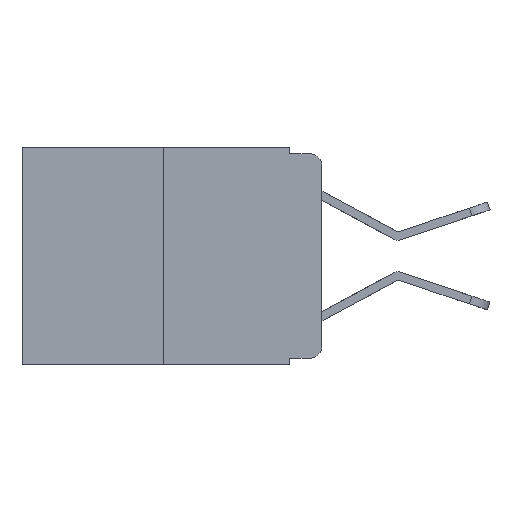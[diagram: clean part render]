
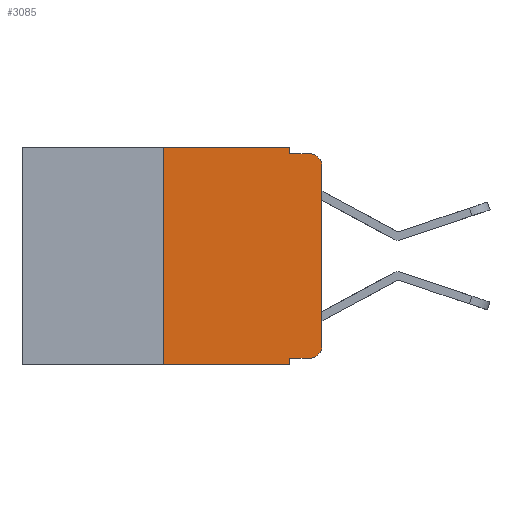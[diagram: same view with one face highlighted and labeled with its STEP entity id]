
A CAD part, left-side view. The second image highlights one B-rep face of the part: STEP entity #3085.
In plain terms, the highlighted planar face has unit normal (-1, 0, 0).
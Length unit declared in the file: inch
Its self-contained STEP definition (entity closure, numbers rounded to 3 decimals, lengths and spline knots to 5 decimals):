
#28 = VERTEX_POINT ( 'NONE', #774 ) ;
#284 = VECTOR ( 'NONE', #11346, 39.37008 ) ;
#288 = CARTESIAN_POINT ( 'NONE',  ( 0., 0.051, 0. ) ) ;
#741 = DIRECTION ( 'NONE',  ( 0., 0., 1. ) ) ;
#774 = CARTESIAN_POINT ( 'NONE',  ( 0., 0.051, 0. ) ) ;
#978 = CARTESIAN_POINT ( 'NONE',  ( 0., 0., -0.03 ) ) ;
#1115 = CARTESIAN_POINT ( 'NONE',  ( 0., 0.02, -0.333 ) ) ;
#1188 = VERTEX_POINT ( 'NONE', #10671 ) ;
#1215 = CARTESIAN_POINT ( 'NONE',  ( 0., 0.051, -0.333 ) ) ;
#1330 = VERTEX_POINT ( 'NONE', #1115 ) ;
#1332 = LINE ( 'NONE', #7927, #8927 ) ;
#1438 = VERTEX_POINT ( 'NONE', #9221 ) ;
#1450 = VERTEX_POINT ( 'NONE', #4686 ) ;
#1580 = EDGE_CURVE ( 'NONE', #1450, #4527, #5750, .T. ) ;
#1722 = AXIS2_PLACEMENT_3D ( 'NONE', #4035, #10585, #5033 ) ;
#1853 = ORIENTED_EDGE ( 'NONE', *, *, #3724, .F. ) ;
#2213 = ORIENTED_EDGE ( 'NONE', *, *, #10275, .T. ) ;
#2307 = EDGE_CURVE ( 'NONE', #28, #1188, #2885, .T. ) ;
#2504 = EDGE_CURVE ( 'NONE', #1450, #8013, #1332, .T. ) ;
#2551 = DIRECTION ( 'NONE',  ( 0., 0., -1. ) ) ;
#2592 = DIRECTION ( 'NONE',  ( 1., 0., 0. ) ) ;
#2665 = VERTEX_POINT ( 'NONE', #11396 ) ;
#2686 = ORIENTED_EDGE ( 'NONE', *, *, #12070, .F. ) ;
#2885 = LINE ( 'NONE', #288, #284 ) ;
#3085 = ADVANCED_FACE ( 'NONE', ( #10567 ), #5547, .F. ) ;
#3231 = CARTESIAN_POINT ( 'NONE',  ( 0., 0.051, 0. ) ) ;
#3233 = CARTESIAN_POINT ( 'NONE',  ( 0., 0.25, 0. ) ) ;
#3294 = ORIENTED_EDGE ( 'NONE', *, *, #2307, .F. ) ;
#3724 = EDGE_CURVE ( 'NONE', #1188, #1438, #7327, .T. ) ;
#3977 = VECTOR ( 'NONE', #741, 39.37008 ) ;
#4012 = CARTESIAN_POINT ( 'NONE',  ( 0., 0.473, 0. ) ) ;
#4035 = CARTESIAN_POINT ( 'NONE',  ( 0., 0.02, -0.313 ) ) ;
#4527 = VERTEX_POINT ( 'NONE', #4533 ) ;
#4533 = CARTESIAN_POINT ( 'NONE',  ( 0., 0.25, 0. ) ) ;
#4546 = LINE ( 'NONE', #1215, #9278 ) ;
#4592 = DIRECTION ( 'NONE',  ( 0., -1., 0. ) ) ;
#4686 = CARTESIAN_POINT ( 'NONE',  ( 0., 0.25, -0.343 ) ) ;
#4696 = LINE ( 'NONE', #9319, #11775 ) ;
#4878 = DIRECTION ( 'NONE',  ( 0., -1., 0. ) ) ;
#4960 = CARTESIAN_POINT ( 'NONE',  ( 0., 0., 0. ) ) ;
#5033 = DIRECTION ( 'NONE',  ( 0., 0., -1. ) ) ;
#5062 = EDGE_CURVE ( 'NONE', #6580, #1438, #5335, .T. ) ;
#5335 = CIRCLE ( 'NONE', #5743, 0.02 ) ;
#5495 = CIRCLE ( 'NONE', #1722, 0.02 ) ;
#5547 = PLANE ( 'NONE',  #9251 ) ;
#5743 = AXIS2_PLACEMENT_3D ( 'NONE', #8003, #7967, #10916 ) ;
#5750 = LINE ( 'NONE', #3233, #6346 ) ;
#6269 = CARTESIAN_POINT ( 'NONE',  ( 0., 0.051, -0.333 ) ) ;
#6346 = VECTOR ( 'NONE', #7991, 39.37008 ) ;
#6372 = EDGE_CURVE ( 'NONE', #2665, #6580, #11141, .T. ) ;
#6580 = VERTEX_POINT ( 'NONE', #978 ) ;
#7327 = LINE ( 'NONE', #12593, #7898 ) ;
#7340 = EDGE_LOOP ( 'NONE', ( #12009, #8517, #1853, #3294, #7661, #12170, #7346, #2686, #10999, #2213 ) ) ;
#7346 = ORIENTED_EDGE ( 'NONE', *, *, #2504, .T. ) ;
#7661 = ORIENTED_EDGE ( 'NONE', *, *, #10975, .F. ) ;
#7898 = VECTOR ( 'NONE', #4878, 39.37008 ) ;
#7927 = CARTESIAN_POINT ( 'NONE',  ( 0., 0.473, -0.343 ) ) ;
#7967 = DIRECTION ( 'NONE',  ( -1., 0., 0. ) ) ;
#7991 = DIRECTION ( 'NONE',  ( 0., 0., 1. ) ) ;
#8003 = CARTESIAN_POINT ( 'NONE',  ( 0., 0.02, -0.03 ) ) ;
#8013 = VERTEX_POINT ( 'NONE', #8109 ) ;
#8109 = CARTESIAN_POINT ( 'NONE',  ( 0., 0.051, -0.343 ) ) ;
#8517 = ORIENTED_EDGE ( 'NONE', *, *, #5062, .T. ) ;
#8927 = VECTOR ( 'NONE', #4592, 39.37008 ) ;
#9221 = CARTESIAN_POINT ( 'NONE',  ( 0., 0.02, -0.01 ) ) ;
#9223 = VERTEX_POINT ( 'NONE', #6269 ) ;
#9251 = AXIS2_PLACEMENT_3D ( 'NONE', #4012, #2592, #2551 ) ;
#9278 = VECTOR ( 'NONE', #11836, 39.37008 ) ;
#9319 = CARTESIAN_POINT ( 'NONE',  ( 0., 0.473, 0. ) ) ;
#9903 = DIRECTION ( 'NONE',  ( 0., 0., -1. ) ) ;
#10192 = DIRECTION ( 'NONE',  ( 0., -1., 0. ) ) ;
#10275 = EDGE_CURVE ( 'NONE', #1330, #2665, #5495, .T. ) ;
#10567 = FACE_OUTER_BOUND ( 'NONE', #7340, .T. ) ;
#10585 = DIRECTION ( 'NONE',  ( -1., 0., 0. ) ) ;
#10671 = CARTESIAN_POINT ( 'NONE',  ( 0., 0.051, -0.01 ) ) ;
#10916 = DIRECTION ( 'NONE',  ( 0., 0., -1. ) ) ;
#10975 = EDGE_CURVE ( 'NONE', #4527, #28, #4696, .T. ) ;
#10999 = ORIENTED_EDGE ( 'NONE', *, *, #11467, .T. ) ;
#11141 = LINE ( 'NONE', #4960, #3977 ) ;
#11346 = DIRECTION ( 'NONE',  ( 0., 0., -1. ) ) ;
#11396 = CARTESIAN_POINT ( 'NONE',  ( 0., 0., -0.313 ) ) ;
#11467 = EDGE_CURVE ( 'NONE', #9223, #1330, #4546, .T. ) ;
#11763 = LINE ( 'NONE', #3231, #12032 ) ;
#11775 = VECTOR ( 'NONE', #10192, 39.37008 ) ;
#11836 = DIRECTION ( 'NONE',  ( 0., -1., 0. ) ) ;
#12009 = ORIENTED_EDGE ( 'NONE', *, *, #6372, .T. ) ;
#12032 = VECTOR ( 'NONE', #9903, 39.37008 ) ;
#12070 = EDGE_CURVE ( 'NONE', #9223, #8013, #11763, .T. ) ;
#12170 = ORIENTED_EDGE ( 'NONE', *, *, #1580, .F. ) ;
#12593 = CARTESIAN_POINT ( 'NONE',  ( 0., 0.051, -0.01 ) ) ;
